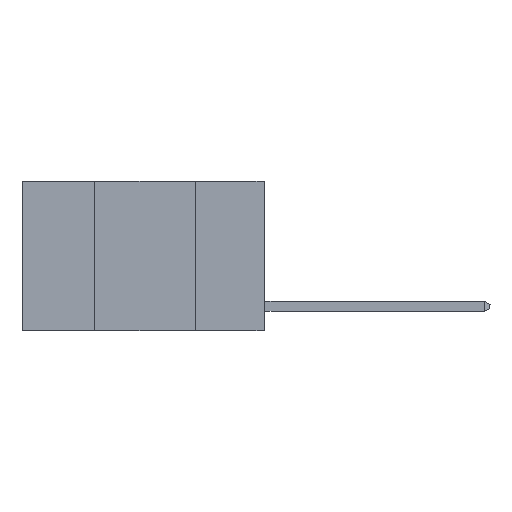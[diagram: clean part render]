
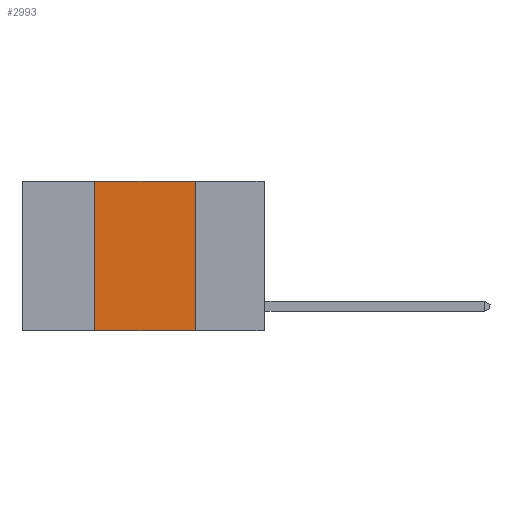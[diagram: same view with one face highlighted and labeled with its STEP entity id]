
A CAD part, left-side view. The second image highlights one B-rep face of the part: STEP entity #2993.
In plain terms, the highlighted planar face has unit normal (-1, 0, 0).
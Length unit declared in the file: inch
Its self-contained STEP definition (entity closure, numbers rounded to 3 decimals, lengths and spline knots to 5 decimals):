
#353 = DIRECTION ( 'NONE',  ( 0., -1., 0. ) ) ;
#1670 = CARTESIAN_POINT ( 'NONE',  ( 0., 0.6, -0.37 ) ) ;
#2104 = EDGE_CURVE ( 'NONE', #10805, #11493, #13228, .T. ) ;
#2176 = AXIS2_PLACEMENT_3D ( 'NONE', #6263, #7459, #8984 ) ;
#2807 = EDGE_LOOP ( 'NONE', ( #9010, #7737, #10167, #12421 ) ) ;
#2857 = VECTOR ( 'NONE', #353, 39.37008 ) ;
#2993 = ADVANCED_FACE ( 'NONE', ( #10781 ), #14605, .F. ) ;
#4091 = CARTESIAN_POINT ( 'NONE',  ( 0., 0.42, -0.37 ) ) ;
#4546 = VERTEX_POINT ( 'NONE', #13055 ) ;
#4590 = VECTOR ( 'NONE', #9607, 39.37008 ) ;
#4760 = CARTESIAN_POINT ( 'NONE',  ( 0., 0.6, 0. ) ) ;
#5550 = EDGE_CURVE ( 'NONE', #15641, #4546, #9395, .T. ) ;
#6030 = DIRECTION ( 'NONE',  ( 0., -1., 0. ) ) ;
#6263 = CARTESIAN_POINT ( 'NONE',  ( 0., 0.6, 0. ) ) ;
#6389 = EDGE_CURVE ( 'NONE', #15641, #10805, #14203, .T. ) ;
#7459 = DIRECTION ( 'NONE',  ( 1., 0., 0. ) ) ;
#7737 = ORIENTED_EDGE ( 'NONE', *, *, #2104, .F. ) ;
#8002 = EDGE_CURVE ( 'NONE', #11493, #4546, #8710, .T. ) ;
#8414 = CARTESIAN_POINT ( 'NONE',  ( 0., 0.42, 0. ) ) ;
#8710 = LINE ( 'NONE', #11728, #14672 ) ;
#8984 = DIRECTION ( 'NONE',  ( 0., 0., -1. ) ) ;
#9008 = CARTESIAN_POINT ( 'NONE',  ( 0., 0.42, 0. ) ) ;
#9010 = ORIENTED_EDGE ( 'NONE', *, *, #8002, .F. ) ;
#9395 = LINE ( 'NONE', #1670, #2857 ) ;
#9607 = DIRECTION ( 'NONE',  ( 0., 0., 1. ) ) ;
#10062 = VECTOR ( 'NONE', #6030, 39.37008 ) ;
#10167 = ORIENTED_EDGE ( 'NONE', *, *, #6389, .F. ) ;
#10781 = FACE_OUTER_BOUND ( 'NONE', #2807, .T. ) ;
#10805 = VERTEX_POINT ( 'NONE', #9008 ) ;
#11493 = VERTEX_POINT ( 'NONE', #14645 ) ;
#11728 = CARTESIAN_POINT ( 'NONE',  ( 0., 0.17, 0. ) ) ;
#12421 = ORIENTED_EDGE ( 'NONE', *, *, #5550, .T. ) ;
#12939 = DIRECTION ( 'NONE',  ( 0., 0., -1. ) ) ;
#13055 = CARTESIAN_POINT ( 'NONE',  ( 0., 0.17, -0.37 ) ) ;
#13228 = LINE ( 'NONE', #4760, #10062 ) ;
#14203 = LINE ( 'NONE', #8414, #4590 ) ;
#14605 = PLANE ( 'NONE',  #2176 ) ;
#14645 = CARTESIAN_POINT ( 'NONE',  ( 0., 0.17, 0. ) ) ;
#14672 = VECTOR ( 'NONE', #12939, 39.37008 ) ;
#15641 = VERTEX_POINT ( 'NONE', #4091 ) ;
